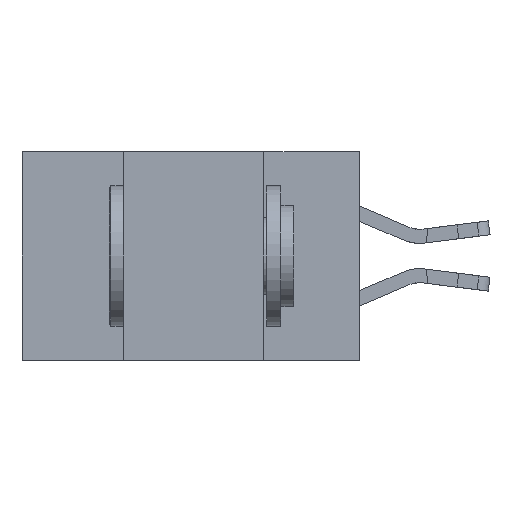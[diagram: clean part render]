
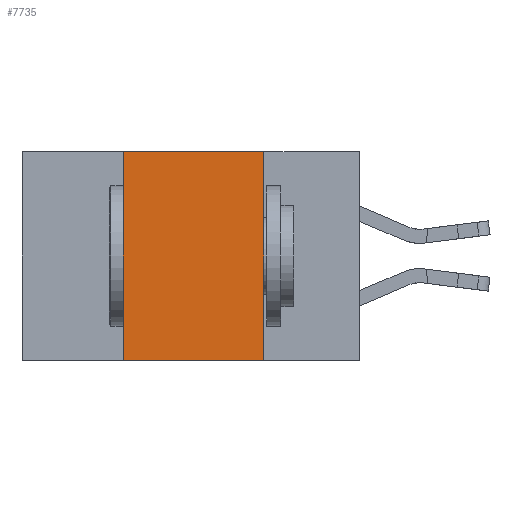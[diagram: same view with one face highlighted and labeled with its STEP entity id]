
A CAD part, left-side view. The second image highlights one B-rep face of the part: STEP entity #7735.
In plain terms, the highlighted planar face has unit normal (-1, 0, 0).
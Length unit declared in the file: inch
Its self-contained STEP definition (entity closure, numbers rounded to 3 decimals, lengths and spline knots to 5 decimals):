
#512 = CARTESIAN_POINT ( 'NONE',  ( 0., 0.42, 0. ) ) ;
#1081 = EDGE_CURVE ( 'NONE', #18791, #11565, #5049, .T. ) ;
#1312 = DIRECTION ( 'NONE',  ( 1., 0., 0. ) ) ;
#4060 = LINE ( 'NONE', #27859, #6477 ) ;
#5049 = LINE ( 'NONE', #512, #9531 ) ;
#6220 = LINE ( 'NONE', #27962, #17229 ) ;
#6477 = VECTOR ( 'NONE', #19126, 39.37008 ) ;
#6496 = DIRECTION ( 'NONE',  ( 0., 0., -1. ) ) ;
#7320 = DIRECTION ( 'NONE',  ( 0., 0., 1. ) ) ;
#7725 = FACE_OUTER_BOUND ( 'NONE', #28365, .T. ) ;
#7735 = ADVANCED_FACE ( 'NONE', ( #7725 ), #20887, .F. ) ;
#7828 = CARTESIAN_POINT ( 'NONE',  ( 0., 0.42, 0. ) ) ;
#8320 = CARTESIAN_POINT ( 'NONE',  ( 0., 0.6, 0. ) ) ;
#9531 = VECTOR ( 'NONE', #7320, 39.37008 ) ;
#10098 = ORIENTED_EDGE ( 'NONE', *, *, #16315, .T. ) ;
#11508 = VERTEX_POINT ( 'NONE', #24598 ) ;
#11565 = VERTEX_POINT ( 'NONE', #7828 ) ;
#12640 = VERTEX_POINT ( 'NONE', #19789 ) ;
#13104 = ORIENTED_EDGE ( 'NONE', *, *, #14228, .F. ) ;
#14228 = EDGE_CURVE ( 'NONE', #12640, #11508, #17931, .T. ) ;
#14981 = DIRECTION ( 'NONE',  ( 0., 0., -1. ) ) ;
#16266 = CARTESIAN_POINT ( 'NONE',  ( 0., 0.42, -0.37 ) ) ;
#16315 = EDGE_CURVE ( 'NONE', #18791, #11508, #4060, .T. ) ;
#17229 = VECTOR ( 'NONE', #28348, 39.37008 ) ;
#17931 = LINE ( 'NONE', #27915, #21363 ) ;
#18791 = VERTEX_POINT ( 'NONE', #16266 ) ;
#19126 = DIRECTION ( 'NONE',  ( 0., -1., 0. ) ) ;
#19789 = CARTESIAN_POINT ( 'NONE',  ( 0., 0.17, 0. ) ) ;
#20887 = PLANE ( 'NONE',  #23234 ) ;
#21096 = ORIENTED_EDGE ( 'NONE', *, *, #25958, .F. ) ;
#21363 = VECTOR ( 'NONE', #14981, 39.37008 ) ;
#23234 = AXIS2_PLACEMENT_3D ( 'NONE', #8320, #1312, #6496 ) ;
#23732 = ORIENTED_EDGE ( 'NONE', *, *, #1081, .F. ) ;
#24598 = CARTESIAN_POINT ( 'NONE',  ( 0., 0.17, -0.37 ) ) ;
#25958 = EDGE_CURVE ( 'NONE', #11565, #12640, #6220, .T. ) ;
#27859 = CARTESIAN_POINT ( 'NONE',  ( 0., 0.6, -0.37 ) ) ;
#27915 = CARTESIAN_POINT ( 'NONE',  ( 0., 0.17, 0. ) ) ;
#27962 = CARTESIAN_POINT ( 'NONE',  ( 0., 0.6, 0. ) ) ;
#28348 = DIRECTION ( 'NONE',  ( 0., -1., 0. ) ) ;
#28365 = EDGE_LOOP ( 'NONE', ( #13104, #21096, #23732, #10098 ) ) ;
